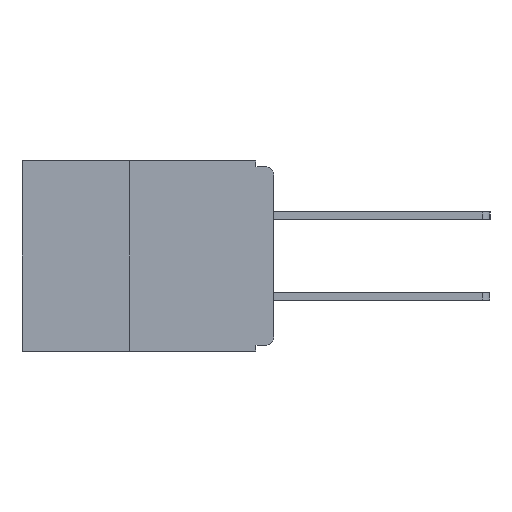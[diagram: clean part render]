
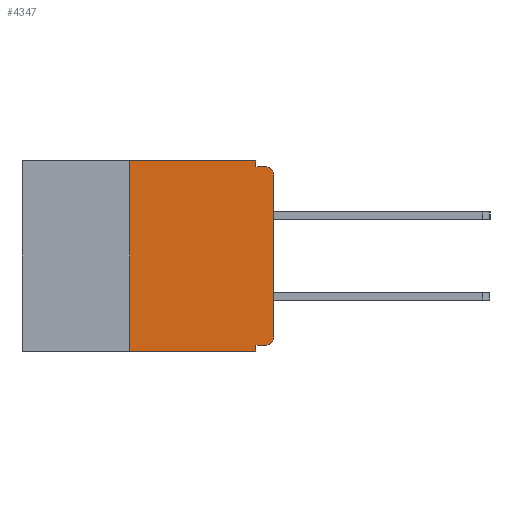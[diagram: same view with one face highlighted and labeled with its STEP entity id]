
A CAD part, left-side view. The second image highlights one B-rep face of the part: STEP entity #4347.
In plain terms, the highlighted planar face has unit normal (-1, 0, 0).
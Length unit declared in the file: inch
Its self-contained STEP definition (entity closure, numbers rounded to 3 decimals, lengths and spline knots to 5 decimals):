
#46 = DIRECTION ( 'NONE',  ( 0., 0., -1. ) ) ;
#140 = CARTESIAN_POINT ( 'NONE',  ( 0., 0.437, 0. ) ) ;
#221 = VERTEX_POINT ( 'NONE', #9402 ) ;
#263 = LINE ( 'NONE', #10445, #13205 ) ;
#303 = CARTESIAN_POINT ( 'NONE',  ( 0., 0.25, -0.33 ) ) ;
#385 = EDGE_LOOP ( 'NONE', ( #1138, #470, #5747, #2571, #1954, #10084, #11507, #13252, #7753, #6759 ) ) ;
#470 = ORIENTED_EDGE ( 'NONE', *, *, #11959, .T. ) ;
#1099 = VERTEX_POINT ( 'NONE', #6825 ) ;
#1138 = ORIENTED_EDGE ( 'NONE', *, *, #7902, .T. ) ;
#1179 = CARTESIAN_POINT ( 'NONE',  ( 0., 0.015, -0.32 ) ) ;
#1655 = AXIS2_PLACEMENT_3D ( 'NONE', #3488, #10897, #4565 ) ;
#1669 = CARTESIAN_POINT ( 'NONE',  ( 0., 0.031, 0. ) ) ;
#1756 = EDGE_CURVE ( 'NONE', #3266, #4899, #263, .T. ) ;
#1762 = LINE ( 'NONE', #4286, #9894 ) ;
#1954 = ORIENTED_EDGE ( 'NONE', *, *, #11460, .F. ) ;
#2239 = CARTESIAN_POINT ( 'NONE',  ( 0., 0.031, -0.01 ) ) ;
#2571 = ORIENTED_EDGE ( 'NONE', *, *, #10298, .F. ) ;
#2667 = DIRECTION ( 'NONE',  ( 0., 0., -1. ) ) ;
#2858 = DIRECTION ( 'NONE',  ( 0., -1., 0. ) ) ;
#2880 = VERTEX_POINT ( 'NONE', #3289 ) ;
#3036 = CARTESIAN_POINT ( 'NONE',  ( 0., 0.031, -0.33 ) ) ;
#3045 = EDGE_CURVE ( 'NONE', #9365, #4899, #10491, .T. ) ;
#3266 = VERTEX_POINT ( 'NONE', #10087 ) ;
#3289 = CARTESIAN_POINT ( 'NONE',  ( 0., 0., -0.305 ) ) ;
#3349 = VERTEX_POINT ( 'NONE', #7944 ) ;
#3488 = CARTESIAN_POINT ( 'NONE',  ( 0., 0.015, -0.305 ) ) ;
#3595 = AXIS2_PLACEMENT_3D ( 'NONE', #140, #11130, #46 ) ;
#4118 = FACE_OUTER_BOUND ( 'NONE', #385, .T. ) ;
#4286 = CARTESIAN_POINT ( 'NONE',  ( 0., 0., -0.32 ) ) ;
#4347 = ADVANCED_FACE ( 'NONE', ( #4118 ), #5409, .F. ) ;
#4549 = DIRECTION ( 'NONE',  ( 0., 0., -1. ) ) ;
#4565 = DIRECTION ( 'NONE',  ( 0., 0., -1. ) ) ;
#4899 = VERTEX_POINT ( 'NONE', #5162 ) ;
#5162 = CARTESIAN_POINT ( 'NONE',  ( 0., 0.031, -0.33 ) ) ;
#5409 = PLANE ( 'NONE',  #3595 ) ;
#5673 = DIRECTION ( 'NONE',  ( -1., 0., 0. ) ) ;
#5706 = VECTOR ( 'NONE', #6621, 39.37008 ) ;
#5747 = ORIENTED_EDGE ( 'NONE', *, *, #10313, .F. ) ;
#5859 = VERTEX_POINT ( 'NONE', #1179 ) ;
#5929 = DIRECTION ( 'NONE',  ( 0., 0., 1. ) ) ;
#6130 = CIRCLE ( 'NONE', #1655, 0.015 ) ;
#6173 = VECTOR ( 'NONE', #9149, 39.37008 ) ;
#6621 = DIRECTION ( 'NONE',  ( 0., 0., 1. ) ) ;
#6759 = ORIENTED_EDGE ( 'NONE', *, *, #13172, .T. ) ;
#6825 = CARTESIAN_POINT ( 'NONE',  ( 0., 0.25, 0. ) ) ;
#7629 = VERTEX_POINT ( 'NONE', #1669 ) ;
#7711 = VECTOR ( 'NONE', #12956, 39.37008 ) ;
#7753 = ORIENTED_EDGE ( 'NONE', *, *, #10777, .F. ) ;
#7902 = EDGE_CURVE ( 'NONE', #2880, #3349, #12309, .T. ) ;
#7944 = CARTESIAN_POINT ( 'NONE',  ( 0., 0., -0.025 ) ) ;
#8050 = VECTOR ( 'NONE', #4549, 39.37008 ) ;
#8348 = CIRCLE ( 'NONE', #11908, 0.015 ) ;
#8556 = LINE ( 'NONE', #303, #5706 ) ;
#8811 = CARTESIAN_POINT ( 'NONE',  ( 0., 0.031, 0. ) ) ;
#9042 = LINE ( 'NONE', #13193, #6173 ) ;
#9111 = CARTESIAN_POINT ( 'NONE',  ( 0., 0., 0. ) ) ;
#9149 = DIRECTION ( 'NONE',  ( 0., -1., 0. ) ) ;
#9365 = VERTEX_POINT ( 'NONE', #12407 ) ;
#9402 = CARTESIAN_POINT ( 'NONE',  ( 0., 0.015, -0.01 ) ) ;
#9620 = VECTOR ( 'NONE', #5929, 39.37008 ) ;
#9677 = DIRECTION ( 'NONE',  ( 0., 1., 0. ) ) ;
#9894 = VECTOR ( 'NONE', #9677, 39.37008 ) ;
#10084 = ORIENTED_EDGE ( 'NONE', *, *, #10892, .F. ) ;
#10087 = CARTESIAN_POINT ( 'NONE',  ( 0., 0.25, -0.33 ) ) ;
#10298 = EDGE_CURVE ( 'NONE', #7629, #10781, #11159, .T. ) ;
#10313 = EDGE_CURVE ( 'NONE', #10781, #221, #10537, .T. ) ;
#10445 = CARTESIAN_POINT ( 'NONE',  ( 0., 0.437, -0.33 ) ) ;
#10491 = LINE ( 'NONE', #3036, #12849 ) ;
#10537 = LINE ( 'NONE', #12912, #7711 ) ;
#10777 = EDGE_CURVE ( 'NONE', #5859, #9365, #1762, .T. ) ;
#10781 = VERTEX_POINT ( 'NONE', #2239 ) ;
#10892 = EDGE_CURVE ( 'NONE', #3266, #1099, #8556, .T. ) ;
#10897 = DIRECTION ( 'NONE',  ( -1., 0., 0. ) ) ;
#11130 = DIRECTION ( 'NONE',  ( 1., 0., 0. ) ) ;
#11159 = LINE ( 'NONE', #8811, #8050 ) ;
#11460 = EDGE_CURVE ( 'NONE', #1099, #7629, #9042, .T. ) ;
#11507 = ORIENTED_EDGE ( 'NONE', *, *, #1756, .T. ) ;
#11908 = AXIS2_PLACEMENT_3D ( 'NONE', #11927, #5673, #12955 ) ;
#11927 = CARTESIAN_POINT ( 'NONE',  ( 0., 0.015, -0.025 ) ) ;
#11959 = EDGE_CURVE ( 'NONE', #3349, #221, #8348, .T. ) ;
#12309 = LINE ( 'NONE', #9111, #9620 ) ;
#12407 = CARTESIAN_POINT ( 'NONE',  ( 0., 0.031, -0.32 ) ) ;
#12849 = VECTOR ( 'NONE', #2667, 39.37008 ) ;
#12912 = CARTESIAN_POINT ( 'NONE',  ( 0., 0., -0.01 ) ) ;
#12955 = DIRECTION ( 'NONE',  ( 0., 0., -1. ) ) ;
#12956 = DIRECTION ( 'NONE',  ( 0., -1., 0. ) ) ;
#13172 = EDGE_CURVE ( 'NONE', #5859, #2880, #6130, .T. ) ;
#13193 = CARTESIAN_POINT ( 'NONE',  ( 0., 0.437, 0. ) ) ;
#13205 = VECTOR ( 'NONE', #2858, 39.37008 ) ;
#13252 = ORIENTED_EDGE ( 'NONE', *, *, #3045, .F. ) ;
